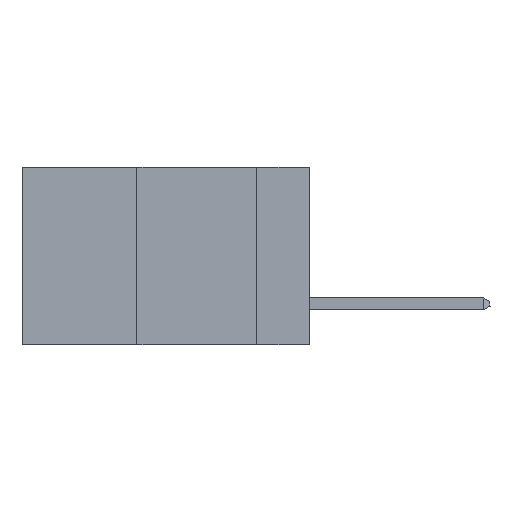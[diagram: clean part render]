
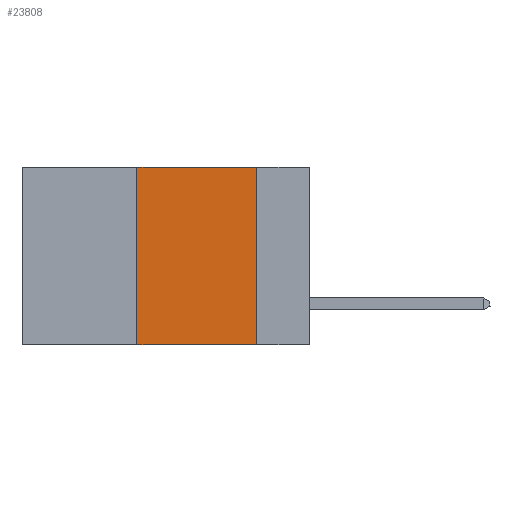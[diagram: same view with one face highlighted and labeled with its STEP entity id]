
A CAD part, left-side view. The second image highlights one B-rep face of the part: STEP entity #23808.
In plain terms, the highlighted planar face has unit normal (-1, 0, 0).
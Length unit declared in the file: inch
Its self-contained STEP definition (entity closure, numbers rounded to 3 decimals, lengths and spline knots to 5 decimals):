
#482 = VERTEX_POINT ( 'NONE', #40944 ) ;
#650 = DIRECTION ( 'NONE',  ( 0., -1., 0. ) ) ;
#1320 = DIRECTION ( 'NONE',  ( 1., 0., 0. ) ) ;
#1615 = CARTESIAN_POINT ( 'NONE',  ( 0., 0.11, 0. ) ) ;
#5000 = DIRECTION ( 'NONE',  ( 0., -1., 0. ) ) ;
#5294 = EDGE_CURVE ( 'NONE', #5790, #33021, #27285, .T. ) ;
#5790 = VERTEX_POINT ( 'NONE', #27939 ) ;
#7073 = CARTESIAN_POINT ( 'NONE',  ( 0., 0.36, -0.37 ) ) ;
#9403 = CARTESIAN_POINT ( 'NONE',  ( 0., 0.6, -0.37 ) ) ;
#9761 = LINE ( 'NONE', #9403, #11485 ) ;
#11485 = VECTOR ( 'NONE', #5000, 39.37008 ) ;
#18334 = EDGE_CURVE ( 'NONE', #482, #5790, #35524, .T. ) ;
#19476 = VERTEX_POINT ( 'NONE', #7073 ) ;
#21874 = VECTOR ( 'NONE', #46142, 39.37008 ) ;
#23808 = ADVANCED_FACE ( 'NONE', ( #25014 ), #41544, .F. ) ;
#24172 = AXIS2_PLACEMENT_3D ( 'NONE', #30427, #1320, #27282 ) ;
#25014 = FACE_OUTER_BOUND ( 'NONE', #30039, .T. ) ;
#25582 = VECTOR ( 'NONE', #650, 39.37008 ) ;
#25756 = EDGE_CURVE ( 'NONE', #19476, #482, #31846, .T. ) ;
#27072 = CARTESIAN_POINT ( 'NONE',  ( 0., 0.6, 0. ) ) ;
#27282 = DIRECTION ( 'NONE',  ( 0., 0., -1. ) ) ;
#27285 = LINE ( 'NONE', #1615, #29029 ) ;
#27939 = CARTESIAN_POINT ( 'NONE',  ( 0., 0.11, 0. ) ) ;
#29029 = VECTOR ( 'NONE', #35751, 39.37008 ) ;
#30039 = EDGE_LOOP ( 'NONE', ( #37099, #44473, #35715, #44974 ) ) ;
#30427 = CARTESIAN_POINT ( 'NONE',  ( 0., 0.6, 0. ) ) ;
#31846 = LINE ( 'NONE', #42308, #21874 ) ;
#33021 = VERTEX_POINT ( 'NONE', #47160 ) ;
#35524 = LINE ( 'NONE', #27072, #25582 ) ;
#35715 = ORIENTED_EDGE ( 'NONE', *, *, #25756, .F. ) ;
#35751 = DIRECTION ( 'NONE',  ( 0., 0., -1. ) ) ;
#37099 = ORIENTED_EDGE ( 'NONE', *, *, #5294, .F. ) ;
#40944 = CARTESIAN_POINT ( 'NONE',  ( 0., 0.36, 0. ) ) ;
#41544 = PLANE ( 'NONE',  #24172 ) ;
#42308 = CARTESIAN_POINT ( 'NONE',  ( 0., 0.36, 0. ) ) ;
#43630 = EDGE_CURVE ( 'NONE', #19476, #33021, #9761, .T. ) ;
#44473 = ORIENTED_EDGE ( 'NONE', *, *, #18334, .F. ) ;
#44974 = ORIENTED_EDGE ( 'NONE', *, *, #43630, .T. ) ;
#46142 = DIRECTION ( 'NONE',  ( 0., 0., 1. ) ) ;
#47160 = CARTESIAN_POINT ( 'NONE',  ( 0., 0.11, -0.37 ) ) ;
